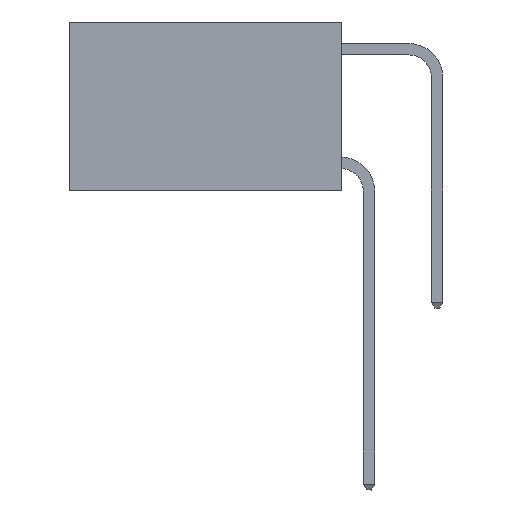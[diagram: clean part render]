
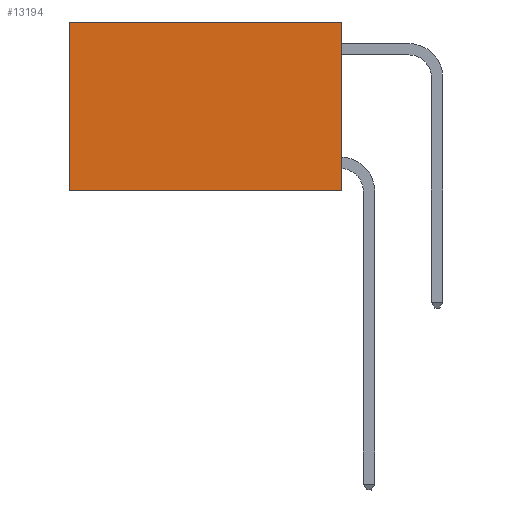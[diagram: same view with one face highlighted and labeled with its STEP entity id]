
A CAD part, left-side view. The second image highlights one B-rep face of the part: STEP entity #13194.
In plain terms, the highlighted planar face has unit normal (-1, 0, 0).
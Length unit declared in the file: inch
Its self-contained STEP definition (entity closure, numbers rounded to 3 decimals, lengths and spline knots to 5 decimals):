
#519 = PLANE ( 'NONE',  #22869 ) ;
#816 = CARTESIAN_POINT ( 'NONE',  ( 0.2625, 0.6, 0. ) ) ;
#1588 = CARTESIAN_POINT ( 'NONE',  ( 0.2625, 0., 0. ) ) ;
#2654 = FACE_OUTER_BOUND ( 'NONE', #19096, .T. ) ;
#2671 = DIRECTION ( 'NONE',  ( 0., 0., -1. ) ) ;
#2756 = CARTESIAN_POINT ( 'NONE',  ( 0.2625, 0., -0.37 ) ) ;
#3559 = CARTESIAN_POINT ( 'NONE',  ( 0.2625, 0.6, -0.37 ) ) ;
#3676 = EDGE_CURVE ( 'NONE', #3759, #16890, #13008, .T. ) ;
#3759 = VERTEX_POINT ( 'NONE', #6835 ) ;
#4267 = VECTOR ( 'NONE', #8728, 39.37008 ) ;
#4473 = CARTESIAN_POINT ( 'NONE',  ( 0.2625, 0., 0. ) ) ;
#6283 = DIRECTION ( 'NONE',  ( 0., 0., -1. ) ) ;
#6712 = ORIENTED_EDGE ( 'NONE', *, *, #14186, .F. ) ;
#6835 = CARTESIAN_POINT ( 'NONE',  ( 0.2625, 0.6, 0. ) ) ;
#8728 = DIRECTION ( 'NONE',  ( 0., 1., 0. ) ) ;
#10083 = VERTEX_POINT ( 'NONE', #2756 ) ;
#10090 = DIRECTION ( 'NONE',  ( 0., 0., -1. ) ) ;
#10490 = LINE ( 'NONE', #12456, #15825 ) ;
#10539 = CARTESIAN_POINT ( 'NONE',  ( 0.2625, 0., 0. ) ) ;
#12376 = DIRECTION ( 'NONE',  ( 0., 1., 0. ) ) ;
#12456 = CARTESIAN_POINT ( 'NONE',  ( 0.2625, 0., -0.37 ) ) ;
#13008 = LINE ( 'NONE', #816, #13539 ) ;
#13071 = LINE ( 'NONE', #22580, #22034 ) ;
#13194 = ADVANCED_FACE ( 'NONE', ( #2654 ), #519, .F. ) ;
#13539 = VECTOR ( 'NONE', #2671, 39.37008 ) ;
#14186 = EDGE_CURVE ( 'NONE', #10083, #16890, #10490, .T. ) ;
#15487 = ORIENTED_EDGE ( 'NONE', *, *, #23130, .T. ) ;
#15825 = VECTOR ( 'NONE', #12376, 39.37008 ) ;
#16890 = VERTEX_POINT ( 'NONE', #3559 ) ;
#17038 = DIRECTION ( 'NONE',  ( 1., 0., 0. ) ) ;
#18577 = LINE ( 'NONE', #10539, #4267 ) ;
#19096 = EDGE_LOOP ( 'NONE', ( #20941, #6712, #19533, #15487 ) ) ;
#19421 = EDGE_CURVE ( 'NONE', #22465, #10083, #13071, .T. ) ;
#19533 = ORIENTED_EDGE ( 'NONE', *, *, #19421, .F. ) ;
#20941 = ORIENTED_EDGE ( 'NONE', *, *, #3676, .T. ) ;
#22034 = VECTOR ( 'NONE', #10090, 39.37008 ) ;
#22465 = VERTEX_POINT ( 'NONE', #1588 ) ;
#22580 = CARTESIAN_POINT ( 'NONE',  ( 0.2625, 0., 0. ) ) ;
#22869 = AXIS2_PLACEMENT_3D ( 'NONE', #4473, #17038, #6283 ) ;
#23130 = EDGE_CURVE ( 'NONE', #22465, #3759, #18577, .T. ) ;
